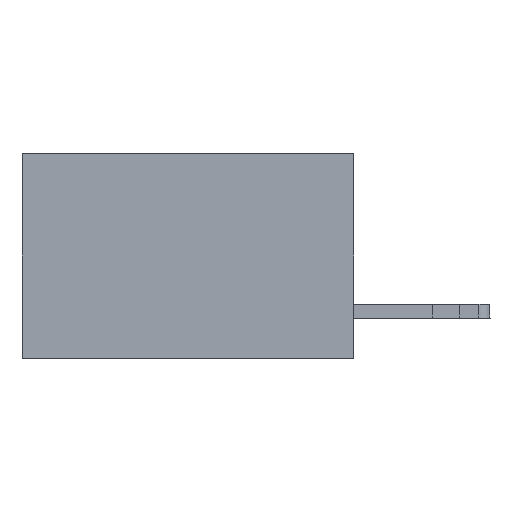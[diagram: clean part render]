
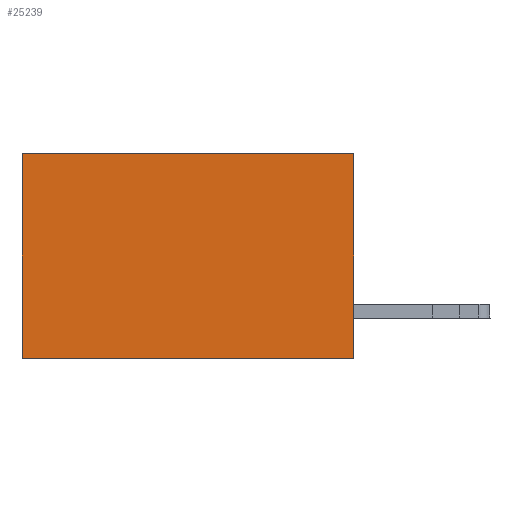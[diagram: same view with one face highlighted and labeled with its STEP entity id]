
A CAD part, left-side view. The second image highlights one B-rep face of the part: STEP entity #25239.
In plain terms, the highlighted planar face has unit normal (-1, 0, 0).
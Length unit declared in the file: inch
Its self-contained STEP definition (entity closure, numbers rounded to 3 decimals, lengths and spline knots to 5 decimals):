
#187 = CARTESIAN_POINT ( 'NONE',  ( 0.2875, 0., 0. ) ) ;
#932 = ORIENTED_EDGE ( 'NONE', *, *, #19520, .T. ) ;
#4324 = ORIENTED_EDGE ( 'NONE', *, *, #5385, .T. ) ;
#5385 = EDGE_CURVE ( 'NONE', #20059, #17305, #6596, .T. ) ;
#5770 = DIRECTION ( 'NONE',  ( 0., 0., -1. ) ) ;
#5909 = LINE ( 'NONE', #14781, #25769 ) ;
#6596 = LINE ( 'NONE', #14177, #13007 ) ;
#6869 = EDGE_LOOP ( 'NONE', ( #4324, #30924, #14343, #932 ) ) ;
#9972 = DIRECTION ( 'NONE',  ( 0., 1., 0. ) ) ;
#13007 = VECTOR ( 'NONE', #22269, 39.37008 ) ;
#13064 = CARTESIAN_POINT ( 'NONE',  ( 0.2875, 0., 0. ) ) ;
#14177 = CARTESIAN_POINT ( 'NONE',  ( 0.2875, 0.6, 0. ) ) ;
#14343 = ORIENTED_EDGE ( 'NONE', *, *, #33298, .F. ) ;
#14781 = CARTESIAN_POINT ( 'NONE',  ( 0.2875, 0., 0. ) ) ;
#15134 = CARTESIAN_POINT ( 'NONE',  ( 0.2875, 0., 0. ) ) ;
#17305 = VERTEX_POINT ( 'NONE', #30066 ) ;
#19274 = PLANE ( 'NONE',  #28130 ) ;
#19520 = EDGE_CURVE ( 'NONE', #23568, #20059, #20171, .T. ) ;
#20059 = VERTEX_POINT ( 'NONE', #27085 ) ;
#20171 = LINE ( 'NONE', #13064, #28131 ) ;
#21828 = VECTOR ( 'NONE', #9972, 39.37008 ) ;
#21959 = DIRECTION ( 'NONE',  ( 1., 0., 0. ) ) ;
#22269 = DIRECTION ( 'NONE',  ( 0., 0., -1. ) ) ;
#23470 = CARTESIAN_POINT ( 'NONE',  ( 0.2875, 0., -0.37 ) ) ;
#23568 = VERTEX_POINT ( 'NONE', #15134 ) ;
#25239 = ADVANCED_FACE ( 'NONE', ( #33997 ), #19274, .F. ) ;
#25769 = VECTOR ( 'NONE', #28260, 39.37008 ) ;
#27085 = CARTESIAN_POINT ( 'NONE',  ( 0.2875, 0.6, 0. ) ) ;
#28110 = LINE ( 'NONE', #34089, #21828 ) ;
#28130 = AXIS2_PLACEMENT_3D ( 'NONE', #187, #21959, #5770 ) ;
#28131 = VECTOR ( 'NONE', #31789, 39.37008 ) ;
#28260 = DIRECTION ( 'NONE',  ( 0., 0., -1. ) ) ;
#30066 = CARTESIAN_POINT ( 'NONE',  ( 0.2875, 0.6, -0.37 ) ) ;
#30099 = EDGE_CURVE ( 'NONE', #30727, #17305, #28110, .T. ) ;
#30727 = VERTEX_POINT ( 'NONE', #23470 ) ;
#30924 = ORIENTED_EDGE ( 'NONE', *, *, #30099, .F. ) ;
#31789 = DIRECTION ( 'NONE',  ( 0., 1., 0. ) ) ;
#33298 = EDGE_CURVE ( 'NONE', #23568, #30727, #5909, .T. ) ;
#33997 = FACE_OUTER_BOUND ( 'NONE', #6869, .T. ) ;
#34089 = CARTESIAN_POINT ( 'NONE',  ( 0.2875, 0., -0.37 ) ) ;
